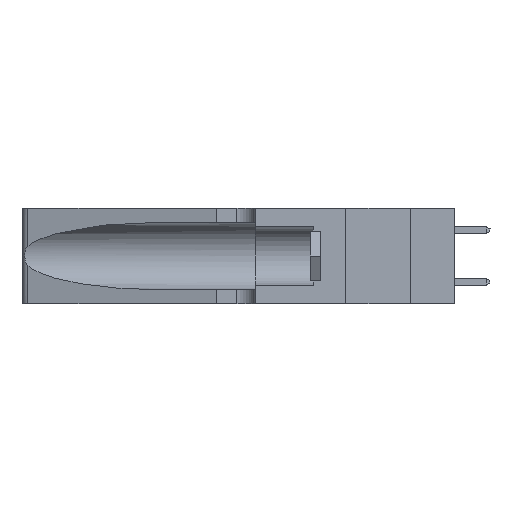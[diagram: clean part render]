
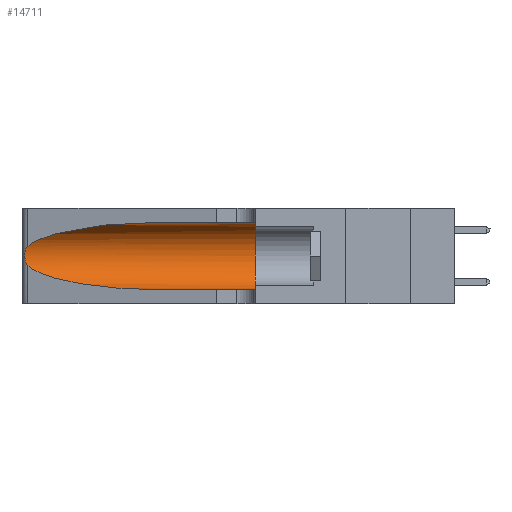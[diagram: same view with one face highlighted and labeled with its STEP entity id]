
A CAD part, left-side view. The second image highlights one B-rep face of the part: STEP entity #14711.
In plain terms, the highlighted cylindrical face has radius 3.308 mm (diameter 6.617 mm), a partial arc.
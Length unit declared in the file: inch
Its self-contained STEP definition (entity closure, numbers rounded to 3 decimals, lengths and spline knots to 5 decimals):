
#20 = EDGE_CURVE ( 'NONE', #17664, #29060, #27798, .T. ) ;
#436 = VERTEX_POINT ( 'NONE', #24654 ) ;
#694 = CARTESIAN_POINT ( 'NONE',  ( 0.25639, 1.23184, 0.21858 ) ) ;
#955 = CARTESIAN_POINT ( 'NONE',  ( 0.25487, 1.22718, 0.22369 ) ) ;
#1167 = ORIENTED_EDGE ( 'NONE', *, *, #31104, .T. ) ;
#1423 = EDGE_CURVE ( 'NONE', #29060, #17029, #8396, .T. ) ;
#3128 = AXIS2_PLACEMENT_3D ( 'NONE', #11396, #14220, #33783 ) ;
#3814 = CARTESIAN_POINT ( 'NONE',  ( 0.25555, 1.22993, 0.14849 ) ) ;
#4144 =( BOUNDED_CURVE ( )  B_SPLINE_CURVE ( 3, ( #17560, #25991, #20037, #14991 ),
 .UNSPECIFIED., .F., .F. ) 
 B_SPLINE_CURVE_WITH_KNOTS ( ( 4, 4 ),
 ( 1.5708, 2.84003 ),
 .UNSPECIFIED. ) 
 CURVE ( )  GEOMETRIC_REPRESENTATION_ITEM ( )  RATIONAL_B_SPLINE_CURVE ( ( 1., 0.87, 0.87, 1. ) ) 
 REPRESENTATION_ITEM ( '' )  );
#4161 = VERTEX_POINT ( 'NONE', #12119 ) ;
#5882 = ORIENTED_EDGE ( 'NONE', *, *, #20, .F. ) ;
#6817 = B_SPLINE_CURVE_WITH_KNOTS ( 'NONE', 3,
 ( #955, #20482, #694, #26340, #23341, #31920, #22981, #9078, #25846, #15086, #14963, #20593, #3814, #31693 ),
 .UNSPECIFIED., .F., .F.,
 ( 4, 2, 2, 2, 2, 2, 4 ),
 ( 0., 0.00027, 0.00053, 0.00107, 0.0016, 0.00187, 0.00214 ),
 .UNSPECIFIED. ) ;
#6820 = CARTESIAN_POINT ( 'NONE',  ( 0.18966, 0.96281, 0.05475 ) ) ;
#7131 = CARTESIAN_POINT ( 'NONE',  ( 0.1305, 0.35, 0.31525 ) ) ;
#7413 = EDGE_LOOP ( 'NONE', ( #1167, #19274, #24436, #11960, #23378, #5882 ) ) ;
#7846 = CARTESIAN_POINT ( 'NONE',  ( 0.1305, 1.61858, 0.05475 ) ) ;
#8396 = CIRCLE ( 'NONE', #3128, 0.13025 ) ;
#9078 = CARTESIAN_POINT ( 'NONE',  ( 0.26075, 1.23896, 0.178 ) ) ;
#10368 = FACE_OUTER_BOUND ( 'NONE', #7413, .T. ) ;
#11396 = CARTESIAN_POINT ( 'NONE',  ( 0.1305, 0.35, 0.185 ) ) ;
#11661 = CYLINDRICAL_SURFACE ( 'NONE', #18202, 0.13025 ) ;
#11889 = VECTOR ( 'NONE', #25345, 39.37008 ) ;
#11960 = ORIENTED_EDGE ( 'NONE', *, *, #27825, .T. ) ;
#12119 = CARTESIAN_POINT ( 'NONE',  ( 0.25487, 1.22718, 0.14631 ) ) ;
#13177 = CARTESIAN_POINT ( 'NONE',  ( 0.1305, 0.72297, 0.31525 ) ) ;
#14220 = DIRECTION ( 'NONE',  ( 0., 1., 0. ) ) ;
#14711 = ADVANCED_FACE ( 'NONE', ( #10368 ), #11661, .F. ) ;
#14963 = CARTESIAN_POINT ( 'NONE',  ( 0.25789, 1.23486, 0.15765 ) ) ;
#14991 = CARTESIAN_POINT ( 'NONE',  ( 0.25487, 1.22718, 0.22369 ) ) ;
#15086 = CARTESIAN_POINT ( 'NONE',  ( 0.25856, 1.23593, 0.16098 ) ) ;
#15620 = CARTESIAN_POINT ( 'NONE',  ( 0.1305, 1.61858, 0.185 ) ) ;
#15759 = DIRECTION ( 'NONE',  ( 0., -1., 0. ) ) ;
#15918 = VERTEX_POINT ( 'NONE', #16430 ) ;
#16091 = CARTESIAN_POINT ( 'NONE',  ( 0.1305, 1.61858, 0.31525 ) ) ;
#16336 = CARTESIAN_POINT ( 'NONE',  ( 0.1305, 0.35, 0.05475 ) ) ;
#16430 = CARTESIAN_POINT ( 'NONE',  ( 0.25487, 1.22718, 0.22369 ) ) ;
#17029 = VERTEX_POINT ( 'NONE', #16336 ) ;
#17560 = CARTESIAN_POINT ( 'NONE',  ( 0.1305, 0.72297, 0.31525 ) ) ;
#17664 = VERTEX_POINT ( 'NONE', #13177 ) ;
#18202 = AXIS2_PLACEMENT_3D ( 'NONE', #15620, #15759, #32846 ) ;
#18237 = EDGE_CURVE ( 'NONE', #15918, #4161, #6817, .T. ) ;
#18786 =( BOUNDED_CURVE ( )  B_SPLINE_CURVE ( 3, ( #29284, #32150, #6820, #30055 ),
 .UNSPECIFIED., .F., .T. ) 
 B_SPLINE_CURVE_WITH_KNOTS ( ( 4, 4 ),
 ( 3.44316, 4.71239 ),
 .UNSPECIFIED. ) 
 CURVE ( )  GEOMETRIC_REPRESENTATION_ITEM ( )  RATIONAL_B_SPLINE_CURVE ( ( 1., 0.87, 0.87, 1. ) ) 
 REPRESENTATION_ITEM ( '' )  );
#19274 = ORIENTED_EDGE ( 'NONE', *, *, #18237, .T. ) ;
#20037 = CARTESIAN_POINT ( 'NONE',  ( 0.2373, 1.15595, 0.28018 ) ) ;
#20482 = CARTESIAN_POINT ( 'NONE',  ( 0.25555, 1.22994, 0.2215 ) ) ;
#20593 = CARTESIAN_POINT ( 'NONE',  ( 0.25639, 1.23186, 0.15144 ) ) ;
#21369 = VECTOR ( 'NONE', #27828, 39.37008 ) ;
#22981 = CARTESIAN_POINT ( 'NONE',  ( 0.26075, 1.23896, 0.19203 ) ) ;
#23341 = CARTESIAN_POINT ( 'NONE',  ( 0.25854, 1.2359, 0.20912 ) ) ;
#23378 = ORIENTED_EDGE ( 'NONE', *, *, #1423, .F. ) ;
#24436 = ORIENTED_EDGE ( 'NONE', *, *, #34486, .T. ) ;
#24654 = CARTESIAN_POINT ( 'NONE',  ( 0.1305, 0.72297, 0.05475 ) ) ;
#25345 = DIRECTION ( 'NONE',  ( 0., -1., 0. ) ) ;
#25846 = CARTESIAN_POINT ( 'NONE',  ( 0.26017, 1.23833, 0.17102 ) ) ;
#25991 = CARTESIAN_POINT ( 'NONE',  ( 0.18966, 0.96281, 0.31525 ) ) ;
#26340 = CARTESIAN_POINT ( 'NONE',  ( 0.25787, 1.23484, 0.2124 ) ) ;
#27798 = LINE ( 'NONE', #16091, #11889 ) ;
#27825 = EDGE_CURVE ( 'NONE', #436, #17029, #31662, .T. ) ;
#27828 = DIRECTION ( 'NONE',  ( 0., -1., 0. ) ) ;
#29060 = VERTEX_POINT ( 'NONE', #7131 ) ;
#29284 = CARTESIAN_POINT ( 'NONE',  ( 0.25487, 1.22718, 0.14631 ) ) ;
#30055 = CARTESIAN_POINT ( 'NONE',  ( 0.1305, 0.72297, 0.05475 ) ) ;
#31104 = EDGE_CURVE ( 'NONE', #17664, #15918, #4144, .T. ) ;
#31662 = LINE ( 'NONE', #7846, #21369 ) ;
#31693 = CARTESIAN_POINT ( 'NONE',  ( 0.25487, 1.22718, 0.14631 ) ) ;
#31920 = CARTESIAN_POINT ( 'NONE',  ( 0.26018, 1.23835, 0.19895 ) ) ;
#32150 = CARTESIAN_POINT ( 'NONE',  ( 0.2373, 1.15595, 0.08982 ) ) ;
#32846 = DIRECTION ( 'NONE',  ( 0., 0., -1. ) ) ;
#33783 = DIRECTION ( 'NONE',  ( 0., 0., 1. ) ) ;
#34486 = EDGE_CURVE ( 'NONE', #4161, #436, #18786, .T. ) ;
